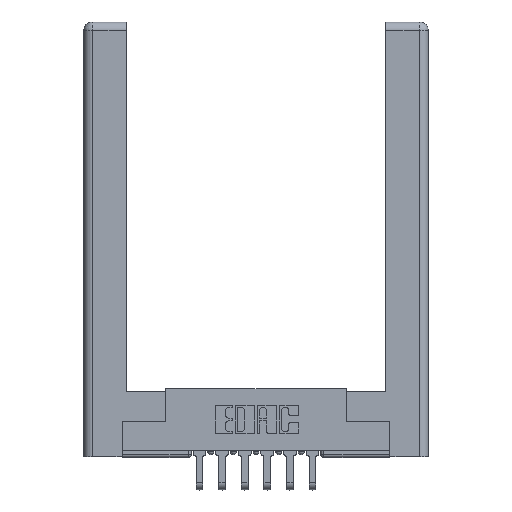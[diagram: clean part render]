
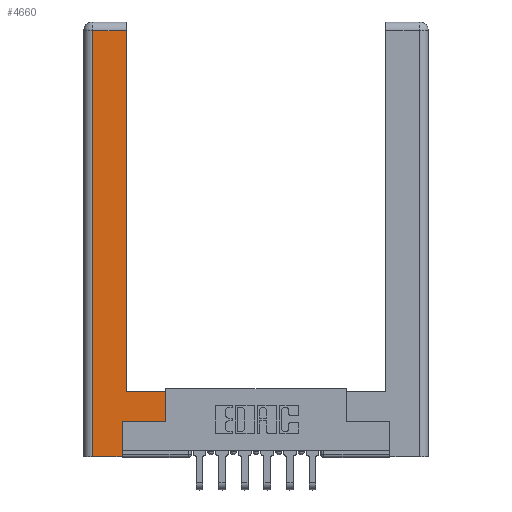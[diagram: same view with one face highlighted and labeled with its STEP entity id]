
A CAD part, top view. The second image highlights one B-rep face of the part: STEP entity #4660.
In plain terms, the highlighted planar face has unit normal (0, 0, 1).
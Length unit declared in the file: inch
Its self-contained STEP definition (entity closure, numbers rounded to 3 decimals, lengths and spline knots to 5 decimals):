
#129 = VERTEX_POINT ( 'NONE', #1782 ) ;
#201 = ORIENTED_EDGE ( 'NONE', *, *, #8436, .T. ) ;
#247 = VECTOR ( 'NONE', #10915, 39.37008 ) ;
#376 = VECTOR ( 'NONE', #9252, 39.37008 ) ;
#485 = CARTESIAN_POINT ( 'NONE',  ( 0.565, 0.45, 0. ) ) ;
#958 = CARTESIAN_POINT ( 'NONE',  ( 0.0615, 0., 0. ) ) ;
#1067 = CARTESIAN_POINT ( 'NONE',  ( 0.265, 0., 0. ) ) ;
#1291 = CARTESIAN_POINT ( 'NONE',  ( 0.265, 0.245, 0. ) ) ;
#1782 = CARTESIAN_POINT ( 'NONE',  ( 0.295, 2.94, 0. ) ) ;
#1982 = CARTESIAN_POINT ( 'NONE',  ( 0.265, 0., 0. ) ) ;
#2010 = LINE ( 'NONE', #958, #12052 ) ;
#2205 = LINE ( 'NONE', #6685, #247 ) ;
#2799 = VERTEX_POINT ( 'NONE', #7275 ) ;
#2967 = VERTEX_POINT ( 'NONE', #13184 ) ;
#3112 = DIRECTION ( 'NONE',  ( 1., 0., 0. ) ) ;
#3461 = VERTEX_POINT ( 'NONE', #11040 ) ;
#3583 = CARTESIAN_POINT ( 'NONE',  ( 0.295, 3., 0. ) ) ;
#3876 = EDGE_CURVE ( 'NONE', #2967, #129, #8785, .T. ) ;
#4124 = DIRECTION ( 'NONE',  ( -1., 0., 0. ) ) ;
#4245 = ORIENTED_EDGE ( 'NONE', *, *, #11060, .T. ) ;
#4299 = LINE ( 'NONE', #1982, #10287 ) ;
#4382 = LINE ( 'NONE', #1291, #10100 ) ;
#4660 = ADVANCED_FACE ( 'NONE', ( #5310 ), #9607, .F. ) ;
#5310 = FACE_OUTER_BOUND ( 'NONE', #10637, .T. ) ;
#5320 = ORIENTED_EDGE ( 'NONE', *, *, #12478, .T. ) ;
#5446 = VERTEX_POINT ( 'NONE', #1067 ) ;
#5628 = CARTESIAN_POINT ( 'NONE',  ( 0.265, 0.245, 0. ) ) ;
#5633 = LINE ( 'NONE', #7739, #12308 ) ;
#5657 = VERTEX_POINT ( 'NONE', #5628 ) ;
#6685 = CARTESIAN_POINT ( 'NONE',  ( 0.295, 0.45, 0. ) ) ;
#6803 = ORIENTED_EDGE ( 'NONE', *, *, #9089, .T. ) ;
#6829 = EDGE_CURVE ( 'NONE', #3461, #5446, #4299, .T. ) ;
#7251 = CARTESIAN_POINT ( 'NONE',  ( 0.0615, 2.94, 0. ) ) ;
#7275 = CARTESIAN_POINT ( 'NONE',  ( 0.565, 0.45, 0. ) ) ;
#7338 = VECTOR ( 'NONE', #12610, 39.37008 ) ;
#7739 = CARTESIAN_POINT ( 'NONE',  ( 0.565, 0.245, 0. ) ) ;
#8123 = EDGE_CURVE ( 'NONE', #9591, #3461, #2010, .T. ) ;
#8319 = LINE ( 'NONE', #7251, #7338 ) ;
#8330 = ORIENTED_EDGE ( 'NONE', *, *, #6829, .T. ) ;
#8436 = EDGE_CURVE ( 'NONE', #129, #9591, #8319, .T. ) ;
#8755 = ORIENTED_EDGE ( 'NONE', *, *, #11044, .T. ) ;
#8785 = LINE ( 'NONE', #3583, #13305 ) ;
#8850 = DIRECTION ( 'NONE',  ( 0., 1., 0. ) ) ;
#9089 = EDGE_CURVE ( 'NONE', #11275, #2799, #11145, .T. ) ;
#9252 = DIRECTION ( 'NONE',  ( 0., 1., 0. ) ) ;
#9591 = VERTEX_POINT ( 'NONE', #11405 ) ;
#9607 = PLANE ( 'NONE',  #10619 ) ;
#10100 = VECTOR ( 'NONE', #12891, 39.37008 ) ;
#10136 = CARTESIAN_POINT ( 'NONE',  ( 0.565, 0.245, 0. ) ) ;
#10287 = VECTOR ( 'NONE', #3112, 39.37008 ) ;
#10619 = AXIS2_PLACEMENT_3D ( 'NONE', #12705, #13828, #4124 ) ;
#10637 = EDGE_LOOP ( 'NONE', ( #13412, #201, #13332, #8330, #4245, #5320, #6803, #8755 ) ) ;
#10915 = DIRECTION ( 'NONE',  ( -1., 0., 0. ) ) ;
#11040 = CARTESIAN_POINT ( 'NONE',  ( 0.0615, 0., 0. ) ) ;
#11044 = EDGE_CURVE ( 'NONE', #2799, #2967, #2205, .T. ) ;
#11060 = EDGE_CURVE ( 'NONE', #5446, #5657, #4382, .T. ) ;
#11145 = LINE ( 'NONE', #485, #376 ) ;
#11275 = VERTEX_POINT ( 'NONE', #10136 ) ;
#11405 = CARTESIAN_POINT ( 'NONE',  ( 0.0615, 2.94, 0. ) ) ;
#12052 = VECTOR ( 'NONE', #13541, 39.37008 ) ;
#12308 = VECTOR ( 'NONE', #13024, 39.37008 ) ;
#12478 = EDGE_CURVE ( 'NONE', #5657, #11275, #5633, .T. ) ;
#12610 = DIRECTION ( 'NONE',  ( -1., 0., 0. ) ) ;
#12705 = CARTESIAN_POINT ( 'NONE',  ( 0., 0., 0. ) ) ;
#12891 = DIRECTION ( 'NONE',  ( 0., 1., 0. ) ) ;
#13024 = DIRECTION ( 'NONE',  ( 1., 0., 0. ) ) ;
#13184 = CARTESIAN_POINT ( 'NONE',  ( 0.295, 0.45, 0. ) ) ;
#13305 = VECTOR ( 'NONE', #8850, 39.37008 ) ;
#13332 = ORIENTED_EDGE ( 'NONE', *, *, #8123, .T. ) ;
#13412 = ORIENTED_EDGE ( 'NONE', *, *, #3876, .T. ) ;
#13541 = DIRECTION ( 'NONE',  ( 0., -1., 0. ) ) ;
#13828 = DIRECTION ( 'NONE',  ( 0., 0., -1. ) ) ;
